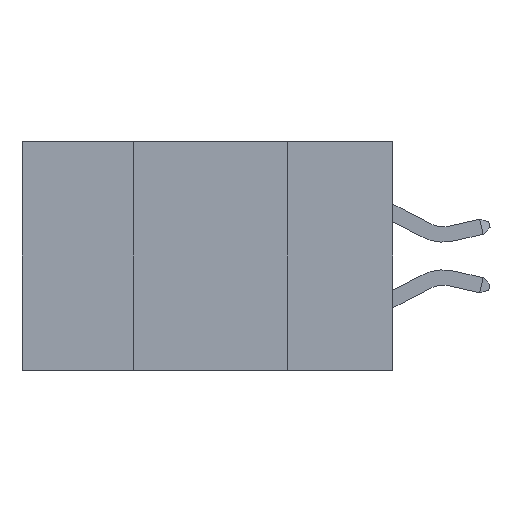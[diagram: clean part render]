
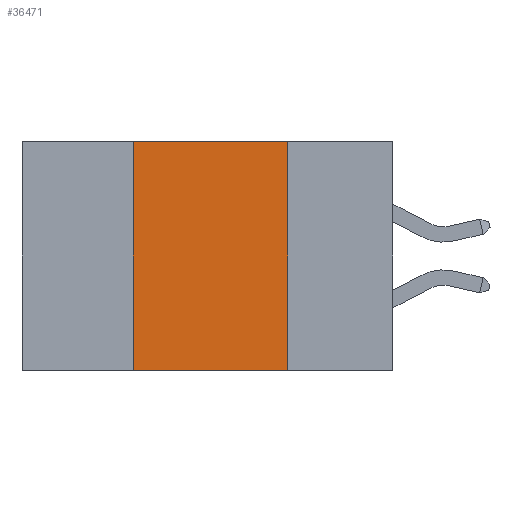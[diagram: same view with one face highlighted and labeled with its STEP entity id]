
A CAD part, left-side view. The second image highlights one B-rep face of the part: STEP entity #36471.
In plain terms, the highlighted planar face has unit normal (-1, 0, 0).
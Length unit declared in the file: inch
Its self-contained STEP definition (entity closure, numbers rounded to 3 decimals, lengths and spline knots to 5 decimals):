
#297 = VERTEX_POINT ( 'NONE', #6796 ) ;
#493 = LINE ( 'NONE', #2717, #32300 ) ;
#2717 = CARTESIAN_POINT ( 'NONE',  ( 0., 0.6, 0. ) ) ;
#2916 = CARTESIAN_POINT ( 'NONE',  ( 0., 0.6, 0. ) ) ;
#3734 = DIRECTION ( 'NONE',  ( 0., 0., -1. ) ) ;
#3866 = VERTEX_POINT ( 'NONE', #20819 ) ;
#6100 = DIRECTION ( 'NONE',  ( 0., 0., -1. ) ) ;
#6428 = ORIENTED_EDGE ( 'NONE', *, *, #33159, .F. ) ;
#6796 = CARTESIAN_POINT ( 'NONE',  ( 0., 0.42, -0.37 ) ) ;
#8024 = VERTEX_POINT ( 'NONE', #26585 ) ;
#10218 = CARTESIAN_POINT ( 'NONE',  ( 0., 0.42, 0. ) ) ;
#11246 = ORIENTED_EDGE ( 'NONE', *, *, #15638, .F. ) ;
#12148 = PLANE ( 'NONE',  #35479 ) ;
#12984 = LINE ( 'NONE', #32469, #35454 ) ;
#13150 = DIRECTION ( 'NONE',  ( 0., 0., 1. ) ) ;
#13763 = ORIENTED_EDGE ( 'NONE', *, *, #16406, .F. ) ;
#13964 = CARTESIAN_POINT ( 'NONE',  ( 0., 0.17, -0.37 ) ) ;
#14489 = EDGE_LOOP ( 'NONE', ( #11246, #6428, #13763, #37561 ) ) ;
#15638 = EDGE_CURVE ( 'NONE', #8024, #28533, #23049, .T. ) ;
#16406 = EDGE_CURVE ( 'NONE', #297, #3866, #19652, .T. ) ;
#17011 = FACE_OUTER_BOUND ( 'NONE', #14489, .T. ) ;
#19652 = LINE ( 'NONE', #10218, #27798 ) ;
#20214 = DIRECTION ( 'NONE',  ( 0., -1., 0. ) ) ;
#20819 = CARTESIAN_POINT ( 'NONE',  ( 0., 0.42, 0. ) ) ;
#23049 = LINE ( 'NONE', #37352, #39162 ) ;
#24533 = DIRECTION ( 'NONE',  ( 1., 0., 0. ) ) ;
#24632 = EDGE_CURVE ( 'NONE', #297, #28533, #12984, .T. ) ;
#26585 = CARTESIAN_POINT ( 'NONE',  ( 0., 0.17, 0. ) ) ;
#27415 = DIRECTION ( 'NONE',  ( 0., -1., 0. ) ) ;
#27798 = VECTOR ( 'NONE', #13150, 39.37008 ) ;
#28533 = VERTEX_POINT ( 'NONE', #13964 ) ;
#32300 = VECTOR ( 'NONE', #27415, 39.37008 ) ;
#32469 = CARTESIAN_POINT ( 'NONE',  ( 0., 0.6, -0.37 ) ) ;
#33159 = EDGE_CURVE ( 'NONE', #3866, #8024, #493, .T. ) ;
#35454 = VECTOR ( 'NONE', #20214, 39.37008 ) ;
#35479 = AXIS2_PLACEMENT_3D ( 'NONE', #2916, #24533, #6100 ) ;
#36471 = ADVANCED_FACE ( 'NONE', ( #17011 ), #12148, .F. ) ;
#37352 = CARTESIAN_POINT ( 'NONE',  ( 0., 0.17, 0. ) ) ;
#37561 = ORIENTED_EDGE ( 'NONE', *, *, #24632, .T. ) ;
#39162 = VECTOR ( 'NONE', #3734, 39.37008 ) ;
